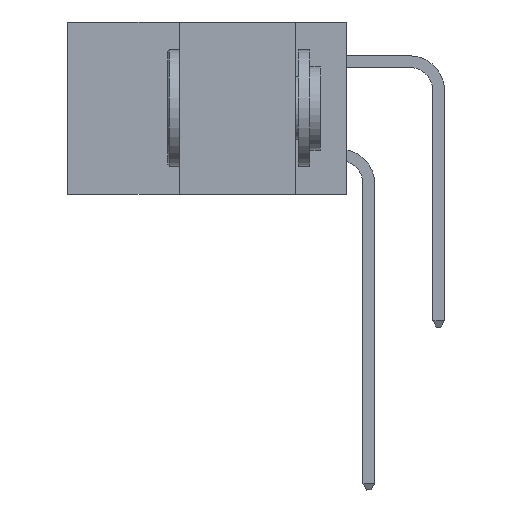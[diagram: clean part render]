
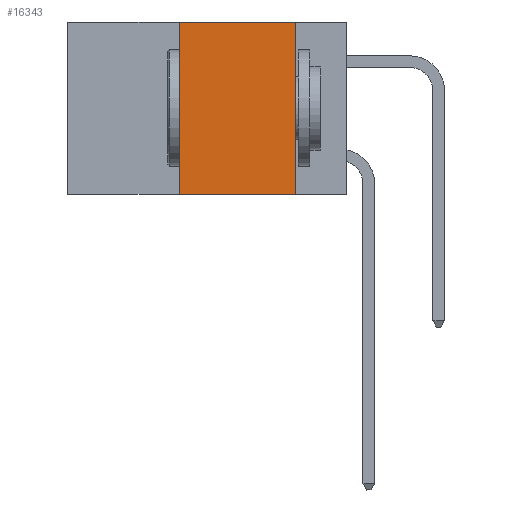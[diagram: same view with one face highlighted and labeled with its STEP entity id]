
A CAD part, left-side view. The second image highlights one B-rep face of the part: STEP entity #16343.
In plain terms, the highlighted planar face has unit normal (-1, 0, 0).
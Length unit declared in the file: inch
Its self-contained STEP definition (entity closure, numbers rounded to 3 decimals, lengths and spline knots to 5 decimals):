
#735 = CARTESIAN_POINT ( 'NONE',  ( 0., 0.36, 0. ) ) ;
#817 = CARTESIAN_POINT ( 'NONE',  ( 0., 0.36, -0.37 ) ) ;
#1998 = VECTOR ( 'NONE', #2158, 39.37008 ) ;
#2158 = DIRECTION ( 'NONE',  ( 0., -1., 0. ) ) ;
#3763 = VERTEX_POINT ( 'NONE', #11102 ) ;
#4478 = CARTESIAN_POINT ( 'NONE',  ( 0., 0.6, -0.37 ) ) ;
#4629 = EDGE_CURVE ( 'NONE', #13617, #3763, #15274, .T. ) ;
#5112 = ORIENTED_EDGE ( 'NONE', *, *, #9056, .F. ) ;
#5392 = VECTOR ( 'NONE', #9156, 39.37008 ) ;
#5489 = EDGE_CURVE ( 'NONE', #5628, #8222, #8632, .T. ) ;
#5628 = VERTEX_POINT ( 'NONE', #817 ) ;
#5646 = CARTESIAN_POINT ( 'NONE',  ( 0., 0.11, 0. ) ) ;
#5797 = LINE ( 'NONE', #5646, #5392 ) ;
#5842 = DIRECTION ( 'NONE',  ( 0., 0., -1. ) ) ;
#6098 = DIRECTION ( 'NONE',  ( 0., 0., 1. ) ) ;
#7981 = ORIENTED_EDGE ( 'NONE', *, *, #11978, .F. ) ;
#8222 = VERTEX_POINT ( 'NONE', #13867 ) ;
#8617 = ORIENTED_EDGE ( 'NONE', *, *, #4629, .F. ) ;
#8632 = LINE ( 'NONE', #4478, #9845 ) ;
#9056 = EDGE_CURVE ( 'NONE', #5628, #13617, #9382, .T. ) ;
#9156 = DIRECTION ( 'NONE',  ( 0., 0., -1. ) ) ;
#9382 = LINE ( 'NONE', #735, #17061 ) ;
#9845 = VECTOR ( 'NONE', #11228, 39.37008 ) ;
#10091 = CARTESIAN_POINT ( 'NONE',  ( 0., 0.6, 0. ) ) ;
#11102 = CARTESIAN_POINT ( 'NONE',  ( 0., 0.11, 0. ) ) ;
#11228 = DIRECTION ( 'NONE',  ( 0., -1., 0. ) ) ;
#11978 = EDGE_CURVE ( 'NONE', #3763, #8222, #5797, .T. ) ;
#12416 = DIRECTION ( 'NONE',  ( 1., 0., 0. ) ) ;
#13506 = CARTESIAN_POINT ( 'NONE',  ( 0., 0.36, 0. ) ) ;
#13617 = VERTEX_POINT ( 'NONE', #13506 ) ;
#13867 = CARTESIAN_POINT ( 'NONE',  ( 0., 0.11, -0.37 ) ) ;
#14013 = ORIENTED_EDGE ( 'NONE', *, *, #5489, .T. ) ;
#15267 = CARTESIAN_POINT ( 'NONE',  ( 0., 0.6, 0. ) ) ;
#15274 = LINE ( 'NONE', #10091, #1998 ) ;
#15752 = FACE_OUTER_BOUND ( 'NONE', #15892, .T. ) ;
#15892 = EDGE_LOOP ( 'NONE', ( #7981, #8617, #5112, #14013 ) ) ;
#16343 = ADVANCED_FACE ( 'NONE', ( #15752 ), #16556, .F. ) ;
#16556 = PLANE ( 'NONE',  #17191 ) ;
#17061 = VECTOR ( 'NONE', #6098, 39.37008 ) ;
#17191 = AXIS2_PLACEMENT_3D ( 'NONE', #15267, #12416, #5842 ) ;
